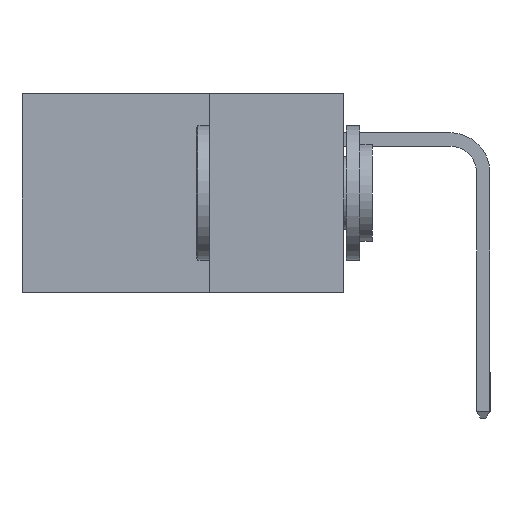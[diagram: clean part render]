
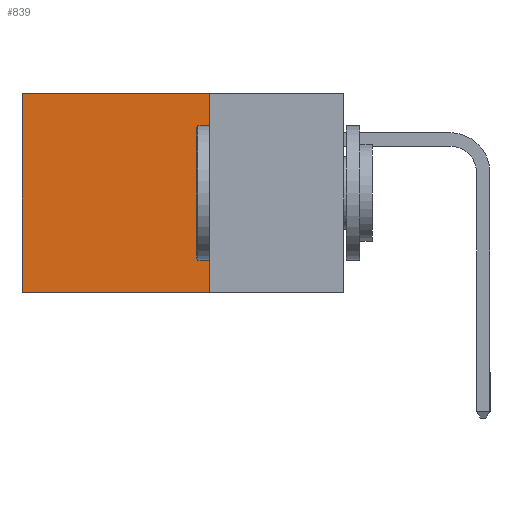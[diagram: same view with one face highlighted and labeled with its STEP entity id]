
A CAD part, left-side view. The second image highlights one B-rep face of the part: STEP entity #839.
In plain terms, the highlighted planar face has unit normal (-1, 0, 0).
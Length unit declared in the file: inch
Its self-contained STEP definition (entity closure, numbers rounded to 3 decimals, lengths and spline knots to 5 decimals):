
#159 = CARTESIAN_POINT ( 'NONE',  ( 0.298, 0.25, 0. ) ) ;
#329 = CARTESIAN_POINT ( 'NONE',  ( 0.298, 0.6, -0.37 ) ) ;
#839 = ADVANCED_FACE ( 'NONE', ( #8870 ), #15551, .F. ) ;
#1523 = EDGE_CURVE ( 'NONE', #20920, #9111, #2572, .T. ) ;
#1594 = DIRECTION ( 'NONE',  ( 0., 1., 0. ) ) ;
#1616 = ORIENTED_EDGE ( 'NONE', *, *, #5946, .F. ) ;
#1648 = EDGE_CURVE ( 'NONE', #9111, #13482, #20764, .T. ) ;
#1819 = VECTOR ( 'NONE', #18365, 39.37008 ) ;
#2241 = DIRECTION ( 'NONE',  ( 0., 0., -1. ) ) ;
#2572 = LINE ( 'NONE', #159, #11965 ) ;
#2707 = CARTESIAN_POINT ( 'NONE',  ( 0.298, 0.6, 0. ) ) ;
#4033 = ORIENTED_EDGE ( 'NONE', *, *, #1648, .T. ) ;
#5946 = EDGE_CURVE ( 'NONE', #20920, #11016, #11628, .T. ) ;
#6030 = CARTESIAN_POINT ( 'NONE',  ( 0.298, 0.25, 0. ) ) ;
#6654 = DIRECTION ( 'NONE',  ( 0., 1., 0. ) ) ;
#7782 = DIRECTION ( 'NONE',  ( 0., 0., -1. ) ) ;
#8870 = FACE_OUTER_BOUND ( 'NONE', #13290, .T. ) ;
#9111 = VERTEX_POINT ( 'NONE', #2707 ) ;
#9142 = CARTESIAN_POINT ( 'NONE',  ( 0.298, 0.25, 0. ) ) ;
#10035 = AXIS2_PLACEMENT_3D ( 'NONE', #9142, #20753, #2241 ) ;
#10327 = VECTOR ( 'NONE', #7782, 39.37008 ) ;
#11016 = VERTEX_POINT ( 'NONE', #21153 ) ;
#11628 = LINE ( 'NONE', #6030, #10327 ) ;
#11965 = VECTOR ( 'NONE', #1594, 39.37008 ) ;
#13290 = EDGE_LOOP ( 'NONE', ( #4033, #21441, #1616, #18927 ) ) ;
#13323 = CARTESIAN_POINT ( 'NONE',  ( 0.298, 0.25, -0.37 ) ) ;
#13482 = VERTEX_POINT ( 'NONE', #329 ) ;
#14853 = CARTESIAN_POINT ( 'NONE',  ( 0.298, 0.6, 0. ) ) ;
#15489 = VECTOR ( 'NONE', #6654, 39.37008 ) ;
#15551 = PLANE ( 'NONE',  #10035 ) ;
#18312 = LINE ( 'NONE', #13323, #15489 ) ;
#18365 = DIRECTION ( 'NONE',  ( 0., 0., -1. ) ) ;
#18927 = ORIENTED_EDGE ( 'NONE', *, *, #1523, .T. ) ;
#20730 = EDGE_CURVE ( 'NONE', #11016, #13482, #18312, .T. ) ;
#20753 = DIRECTION ( 'NONE',  ( 1., 0., 0. ) ) ;
#20764 = LINE ( 'NONE', #14853, #1819 ) ;
#20805 = CARTESIAN_POINT ( 'NONE',  ( 0.298, 0.25, 0. ) ) ;
#20920 = VERTEX_POINT ( 'NONE', #20805 ) ;
#21153 = CARTESIAN_POINT ( 'NONE',  ( 0.298, 0.25, -0.37 ) ) ;
#21441 = ORIENTED_EDGE ( 'NONE', *, *, #20730, .F. ) ;
